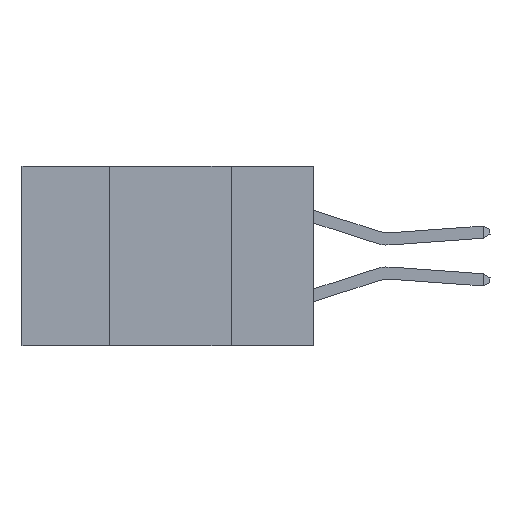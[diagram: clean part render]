
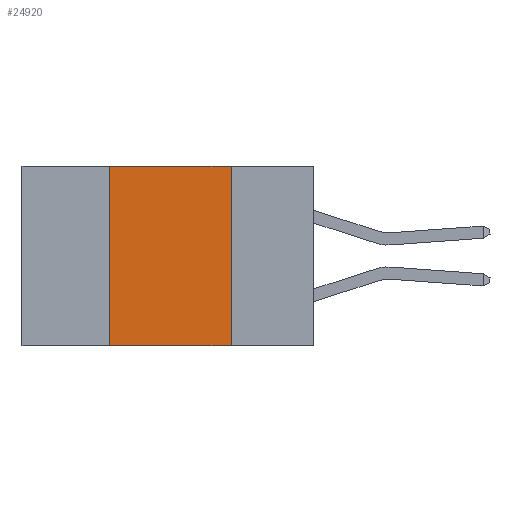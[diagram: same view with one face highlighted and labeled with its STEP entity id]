
A CAD part, left-side view. The second image highlights one B-rep face of the part: STEP entity #24920.
In plain terms, the highlighted planar face has unit normal (-1, 0, 0).
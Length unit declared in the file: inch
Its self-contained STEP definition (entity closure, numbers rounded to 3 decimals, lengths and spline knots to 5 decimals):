
#480 = EDGE_CURVE ( 'NONE', #13455, #27712, #9684, .T. ) ;
#1852 = CARTESIAN_POINT ( 'NONE',  ( 0., 0.6, 0. ) ) ;
#4448 = CARTESIAN_POINT ( 'NONE',  ( 0., 0.42, 0. ) ) ;
#7135 = ORIENTED_EDGE ( 'NONE', *, *, #23624, .T. ) ;
#8569 = CARTESIAN_POINT ( 'NONE',  ( 0., 0.6, 0. ) ) ;
#9445 = CARTESIAN_POINT ( 'NONE',  ( 0., 0.6, -0.37 ) ) ;
#9684 = LINE ( 'NONE', #8569, #11803 ) ;
#10034 = DIRECTION ( 'NONE',  ( 0., 0., -1. ) ) ;
#10100 = VERTEX_POINT ( 'NONE', #12767 ) ;
#10539 = LINE ( 'NONE', #33647, #34775 ) ;
#10798 = ORIENTED_EDGE ( 'NONE', *, *, #480, .F. ) ;
#11803 = VECTOR ( 'NONE', #33051, 39.37008 ) ;
#11805 = CARTESIAN_POINT ( 'NONE',  ( 0., 0.17, 0. ) ) ;
#12056 = DIRECTION ( 'NONE',  ( 0., -1., 0. ) ) ;
#12074 = AXIS2_PLACEMENT_3D ( 'NONE', #1852, #23301, #10034 ) ;
#12365 = DIRECTION ( 'NONE',  ( 0., 0., 1. ) ) ;
#12767 = CARTESIAN_POINT ( 'NONE',  ( 0., 0.42, -0.37 ) ) ;
#13455 = VERTEX_POINT ( 'NONE', #4448 ) ;
#18150 = EDGE_CURVE ( 'NONE', #10100, #13455, #10539, .T. ) ;
#21146 = FACE_OUTER_BOUND ( 'NONE', #33500, .T. ) ;
#22680 = LINE ( 'NONE', #9445, #26086 ) ;
#23301 = DIRECTION ( 'NONE',  ( 1., 0., 0. ) ) ;
#23624 = EDGE_CURVE ( 'NONE', #10100, #30375, #22680, .T. ) ;
#24373 = DIRECTION ( 'NONE',  ( 0., 0., -1. ) ) ;
#24440 = LINE ( 'NONE', #32508, #30442 ) ;
#24920 = ADVANCED_FACE ( 'NONE', ( #21146 ), #31640, .F. ) ;
#26086 = VECTOR ( 'NONE', #12056, 39.37008 ) ;
#26130 = CARTESIAN_POINT ( 'NONE',  ( 0., 0.17, -0.37 ) ) ;
#27712 = VERTEX_POINT ( 'NONE', #11805 ) ;
#30317 = ORIENTED_EDGE ( 'NONE', *, *, #18150, .F. ) ;
#30375 = VERTEX_POINT ( 'NONE', #26130 ) ;
#30442 = VECTOR ( 'NONE', #24373, 39.37008 ) ;
#31640 = PLANE ( 'NONE',  #12074 ) ;
#32508 = CARTESIAN_POINT ( 'NONE',  ( 0., 0.17, 0. ) ) ;
#32679 = EDGE_CURVE ( 'NONE', #27712, #30375, #24440, .T. ) ;
#33051 = DIRECTION ( 'NONE',  ( 0., -1., 0. ) ) ;
#33500 = EDGE_LOOP ( 'NONE', ( #34404, #10798, #30317, #7135 ) ) ;
#33647 = CARTESIAN_POINT ( 'NONE',  ( 0., 0.42, 0. ) ) ;
#34404 = ORIENTED_EDGE ( 'NONE', *, *, #32679, .F. ) ;
#34775 = VECTOR ( 'NONE', #12365, 39.37008 ) ;
